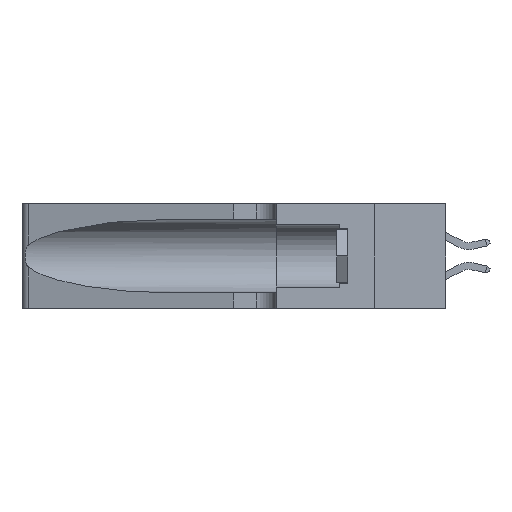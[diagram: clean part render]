
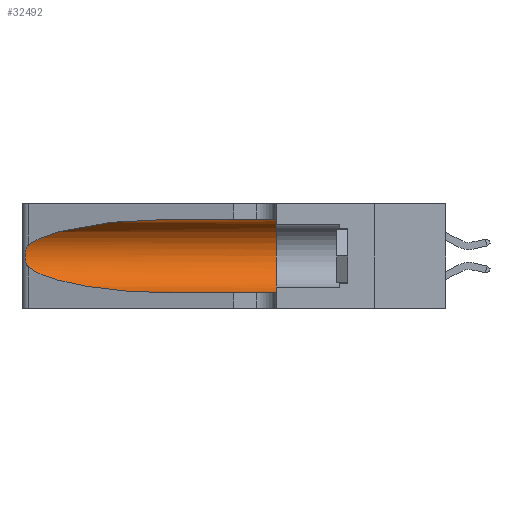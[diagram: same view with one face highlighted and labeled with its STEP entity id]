
A CAD part, left-side view. The second image highlights one B-rep face of the part: STEP entity #32492.
In plain terms, the highlighted cylindrical face has radius 3.308 mm (diameter 6.617 mm), a partial arc.
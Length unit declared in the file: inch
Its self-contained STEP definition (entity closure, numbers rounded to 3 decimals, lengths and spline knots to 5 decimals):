
#118 = VERTEX_POINT ( 'NONE', #35163 ) ;
#624 = VECTOR ( 'NONE', #24159, 39.37008 ) ;
#808 = DIRECTION ( 'NONE',  ( 0., 0., 1. ) ) ;
#924 = CARTESIAN_POINT ( 'NONE',  ( 0.18966, 0.96281, 0.31525 ) ) ;
#1111 = CARTESIAN_POINT ( 'NONE',  ( 0.25639, 1.23186, 0.15144 ) ) ;
#2583 = EDGE_CURVE ( 'NONE', #39753, #19107, #22398, .T. ) ;
#3140 = CARTESIAN_POINT ( 'NONE',  ( 0.25639, 1.23184, 0.21858 ) ) ;
#3183 = CARTESIAN_POINT ( 'NONE',  ( 0.25487, 1.22718, 0.14631 ) ) ;
#4088 = CARTESIAN_POINT ( 'NONE',  ( 0.25555, 1.22993, 0.14849 ) ) ;
#4098 = DIRECTION ( 'NONE',  ( 0., 0., -1. ) ) ;
#7039 = CARTESIAN_POINT ( 'NONE',  ( 0.26017, 1.23833, 0.17102 ) ) ;
#8497 = EDGE_CURVE ( 'NONE', #39753, #17960, #35150, .T. ) ;
#8974 = CIRCLE ( 'NONE', #23977, 0.13025 ) ;
#9353 = CARTESIAN_POINT ( 'NONE',  ( 0.25487, 1.22718, 0.22369 ) ) ;
#9902 = CARTESIAN_POINT ( 'NONE',  ( 0.26018, 1.23835, 0.19895 ) ) ;
#10293 = ORIENTED_EDGE ( 'NONE', *, *, #17634, .T. ) ;
#10306 = CARTESIAN_POINT ( 'NONE',  ( 0.25854, 1.2359, 0.20912 ) ) ;
#10354 = EDGE_CURVE ( 'NONE', #19107, #36391, #18754, .T. ) ;
#11295 = VERTEX_POINT ( 'NONE', #31395 ) ;
#13443 = EDGE_CURVE ( 'NONE', #118, #11295, #14710, .T. ) ;
#13580 = CARTESIAN_POINT ( 'NONE',  ( 0.25856, 1.23593, 0.16098 ) ) ;
#13741 = CARTESIAN_POINT ( 'NONE',  ( 0.1305, 1.61858, 0.185 ) ) ;
#13865 = DIRECTION ( 'NONE',  ( 0., 1., 0. ) ) ;
#14686 = DIRECTION ( 'NONE',  ( 0., -1., 0. ) ) ;
#14710 = LINE ( 'NONE', #40522, #24866 ) ;
#15499 = EDGE_CURVE ( 'NONE', #17960, #11295, #8974, .T. ) ;
#15555 = CARTESIAN_POINT ( 'NONE',  ( 0.2373, 1.15595, 0.28018 ) ) ;
#15588 = CYLINDRICAL_SURFACE ( 'NONE', #31155, 0.13025 ) ;
#15674 = CARTESIAN_POINT ( 'NONE',  ( 0.18966, 0.96281, 0.05475 ) ) ;
#16455 = CARTESIAN_POINT ( 'NONE',  ( 0.26075, 1.23896, 0.178 ) ) ;
#17066 = FACE_OUTER_BOUND ( 'NONE', #18209, .T. ) ;
#17291 = DIRECTION ( 'NONE',  ( 0., -1., 0. ) ) ;
#17432 = CARTESIAN_POINT ( 'NONE',  ( 0.25487, 1.22718, 0.14631 ) ) ;
#17572 = CARTESIAN_POINT ( 'NONE',  ( 0.25487, 1.22718, 0.22369 ) ) ;
#17634 = EDGE_CURVE ( 'NONE', #36391, #118, #31229, .T. ) ;
#17960 = VERTEX_POINT ( 'NONE', #29234 ) ;
#18209 = EDGE_LOOP ( 'NONE', ( #24308, #27755, #10293, #25567, #41026, #39295 ) ) ;
#18754 = B_SPLINE_CURVE_WITH_KNOTS ( 'NONE', 3,
 ( #9353, #35429, #3140, #32474, #10306, #9902, #26516, #16455, #7039, #13580, #20271, #1111, #4088, #17432 ),
 .UNSPECIFIED., .F., .F.,
 ( 4, 2, 2, 2, 2, 2, 4 ),
 ( 0., 0.00027, 0.00053, 0.00107, 0.0016, 0.00187, 0.00214 ),
 .UNSPECIFIED. ) ;
#19107 = VERTEX_POINT ( 'NONE', #25922 ) ;
#20271 = CARTESIAN_POINT ( 'NONE',  ( 0.25789, 1.23486, 0.15765 ) ) ;
#21952 = CARTESIAN_POINT ( 'NONE',  ( 0.1305, 0.72297, 0.31525 ) ) ;
#22398 =( BOUNDED_CURVE ( )  B_SPLINE_CURVE ( 3, ( #30951, #924, #15555, #17572 ),
 .UNSPECIFIED., .F., .F. ) 
 B_SPLINE_CURVE_WITH_KNOTS ( ( 4, 4 ),
 ( 1.5708, 2.84003 ),
 .UNSPECIFIED. ) 
 CURVE ( )  GEOMETRIC_REPRESENTATION_ITEM ( )  RATIONAL_B_SPLINE_CURVE ( ( 1., 0.87, 0.87, 1. ) ) 
 REPRESENTATION_ITEM ( '' )  );
#22500 = CARTESIAN_POINT ( 'NONE',  ( 0.2373, 1.15595, 0.08982 ) ) ;
#23977 = AXIS2_PLACEMENT_3D ( 'NONE', #33145, #13865, #808 ) ;
#24159 = DIRECTION ( 'NONE',  ( 0., -1., 0. ) ) ;
#24308 = ORIENTED_EDGE ( 'NONE', *, *, #2583, .T. ) ;
#24866 = VECTOR ( 'NONE', #14686, 39.37008 ) ;
#25567 = ORIENTED_EDGE ( 'NONE', *, *, #13443, .T. ) ;
#25922 = CARTESIAN_POINT ( 'NONE',  ( 0.25487, 1.22718, 0.22369 ) ) ;
#26516 = CARTESIAN_POINT ( 'NONE',  ( 0.26075, 1.23896, 0.19203 ) ) ;
#27755 = ORIENTED_EDGE ( 'NONE', *, *, #10354, .T. ) ;
#29234 = CARTESIAN_POINT ( 'NONE',  ( 0.1305, 0.35, 0.31525 ) ) ;
#30391 = CARTESIAN_POINT ( 'NONE',  ( 0.1305, 1.61858, 0.31525 ) ) ;
#30951 = CARTESIAN_POINT ( 'NONE',  ( 0.1305, 0.72297, 0.31525 ) ) ;
#31155 = AXIS2_PLACEMENT_3D ( 'NONE', #13741, #17291, #4098 ) ;
#31229 =( BOUNDED_CURVE ( )  B_SPLINE_CURVE ( 3, ( #3183, #22500, #15674, #38286 ),
 .UNSPECIFIED., .F., .F. ) 
 B_SPLINE_CURVE_WITH_KNOTS ( ( 4, 4 ),
 ( 3.44316, 4.71239 ),
 .UNSPECIFIED. ) 
 CURVE ( )  GEOMETRIC_REPRESENTATION_ITEM ( )  RATIONAL_B_SPLINE_CURVE ( ( 1., 0.87, 0.87, 1. ) ) 
 REPRESENTATION_ITEM ( '' )  );
#31395 = CARTESIAN_POINT ( 'NONE',  ( 0.1305, 0.35, 0.05475 ) ) ;
#32474 = CARTESIAN_POINT ( 'NONE',  ( 0.25787, 1.23484, 0.2124 ) ) ;
#32492 = ADVANCED_FACE ( 'NONE', ( #17066 ), #15588, .F. ) ;
#33145 = CARTESIAN_POINT ( 'NONE',  ( 0.1305, 0.35, 0.185 ) ) ;
#35150 = LINE ( 'NONE', #30391, #624 ) ;
#35163 = CARTESIAN_POINT ( 'NONE',  ( 0.1305, 0.72297, 0.05475 ) ) ;
#35429 = CARTESIAN_POINT ( 'NONE',  ( 0.25555, 1.22994, 0.2215 ) ) ;
#36391 = VERTEX_POINT ( 'NONE', #38664 ) ;
#38286 = CARTESIAN_POINT ( 'NONE',  ( 0.1305, 0.72297, 0.05475 ) ) ;
#38664 = CARTESIAN_POINT ( 'NONE',  ( 0.25487, 1.22718, 0.14631 ) ) ;
#39295 = ORIENTED_EDGE ( 'NONE', *, *, #8497, .F. ) ;
#39753 = VERTEX_POINT ( 'NONE', #21952 ) ;
#40522 = CARTESIAN_POINT ( 'NONE',  ( 0.1305, 1.61858, 0.05475 ) ) ;
#41026 = ORIENTED_EDGE ( 'NONE', *, *, #15499, .F. ) ;
